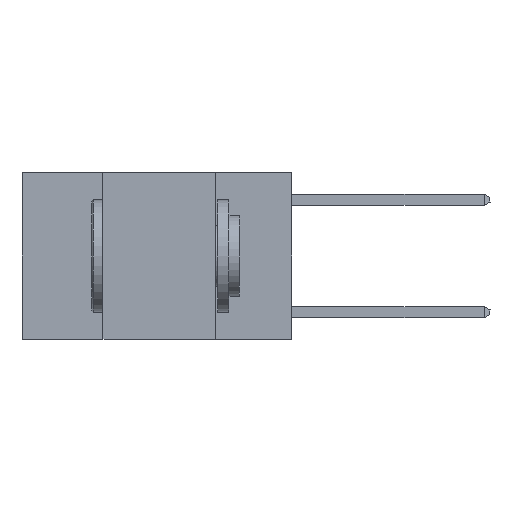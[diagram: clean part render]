
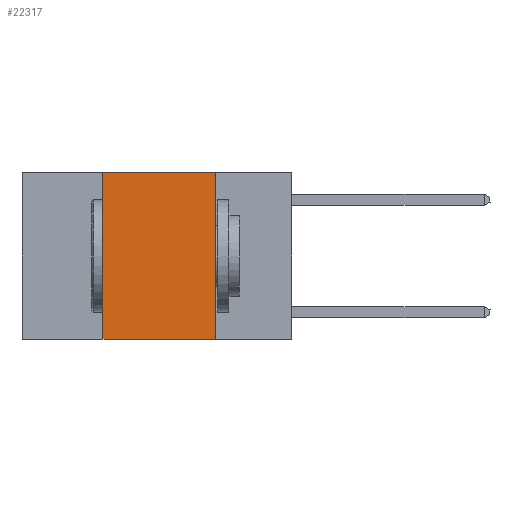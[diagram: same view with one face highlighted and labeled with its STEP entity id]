
A CAD part, left-side view. The second image highlights one B-rep face of the part: STEP entity #22317.
In plain terms, the highlighted planar face has unit normal (-1, 0, 0).
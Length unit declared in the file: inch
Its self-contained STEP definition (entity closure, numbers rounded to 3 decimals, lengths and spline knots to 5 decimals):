
#560 = DIRECTION ( 'NONE',  ( 1., 0., 0. ) ) ;
#567 = CARTESIAN_POINT ( 'NONE',  ( 0., 0.17, -0.37 ) ) ;
#732 = CARTESIAN_POINT ( 'NONE',  ( 0., 0.6, -0.37 ) ) ;
#1087 = ORIENTED_EDGE ( 'NONE', *, *, #9108, .T. ) ;
#3110 = VECTOR ( 'NONE', #22624, 39.37008 ) ;
#3824 = ORIENTED_EDGE ( 'NONE', *, *, #20569, .F. ) ;
#5036 = VERTEX_POINT ( 'NONE', #24522 ) ;
#5765 = DIRECTION ( 'NONE',  ( 0., 0., -1. ) ) ;
#6626 = AXIS2_PLACEMENT_3D ( 'NONE', #7949, #560, #17267 ) ;
#7334 = ORIENTED_EDGE ( 'NONE', *, *, #28068, .F. ) ;
#7337 = VECTOR ( 'NONE', #26602, 39.37008 ) ;
#7351 = LINE ( 'NONE', #27990, #11704 ) ;
#7949 = CARTESIAN_POINT ( 'NONE',  ( 0., 0.6, 0. ) ) ;
#8730 = CARTESIAN_POINT ( 'NONE',  ( 0., 0.42, 0. ) ) ;
#8934 = EDGE_CURVE ( 'NONE', #10437, #5036, #7351, .T. ) ;
#9108 = EDGE_CURVE ( 'NONE', #14786, #14530, #21700, .T. ) ;
#10200 = CARTESIAN_POINT ( 'NONE',  ( 0., 0.17, 0. ) ) ;
#10437 = VERTEX_POINT ( 'NONE', #19457 ) ;
#11279 = CARTESIAN_POINT ( 'NONE',  ( 0., 0.42, -0.37 ) ) ;
#11704 = VECTOR ( 'NONE', #25832, 39.37008 ) ;
#12984 = ORIENTED_EDGE ( 'NONE', *, *, #8934, .F. ) ;
#13461 = LINE ( 'NONE', #8730, #3110 ) ;
#14530 = VERTEX_POINT ( 'NONE', #567 ) ;
#14653 = FACE_OUTER_BOUND ( 'NONE', #20991, .T. ) ;
#14786 = VERTEX_POINT ( 'NONE', #11279 ) ;
#17267 = DIRECTION ( 'NONE',  ( 0., 0., -1. ) ) ;
#19457 = CARTESIAN_POINT ( 'NONE',  ( 0., 0.42, 0. ) ) ;
#20569 = EDGE_CURVE ( 'NONE', #14786, #10437, #13461, .T. ) ;
#20991 = EDGE_LOOP ( 'NONE', ( #7334, #12984, #3824, #1087 ) ) ;
#21438 = VECTOR ( 'NONE', #5765, 39.37008 ) ;
#21700 = LINE ( 'NONE', #732, #7337 ) ;
#22317 = ADVANCED_FACE ( 'NONE', ( #14653 ), #26114, .F. ) ;
#22624 = DIRECTION ( 'NONE',  ( 0., 0., 1. ) ) ;
#24095 = LINE ( 'NONE', #10200, #21438 ) ;
#24522 = CARTESIAN_POINT ( 'NONE',  ( 0., 0.17, 0. ) ) ;
#25832 = DIRECTION ( 'NONE',  ( 0., -1., 0. ) ) ;
#26114 = PLANE ( 'NONE',  #6626 ) ;
#26602 = DIRECTION ( 'NONE',  ( 0., -1., 0. ) ) ;
#27990 = CARTESIAN_POINT ( 'NONE',  ( 0., 0.6, 0. ) ) ;
#28068 = EDGE_CURVE ( 'NONE', #5036, #14530, #24095, .T. ) ;
